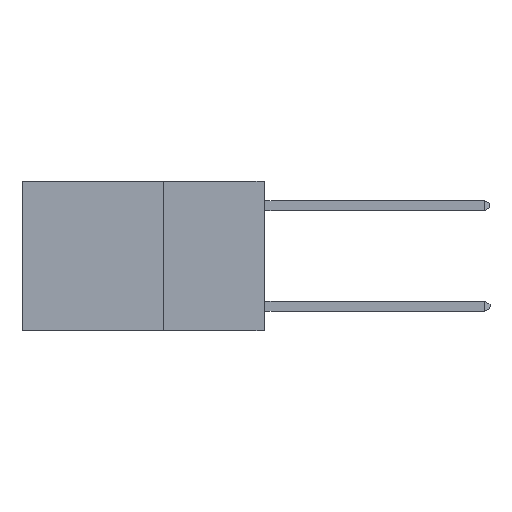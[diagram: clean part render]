
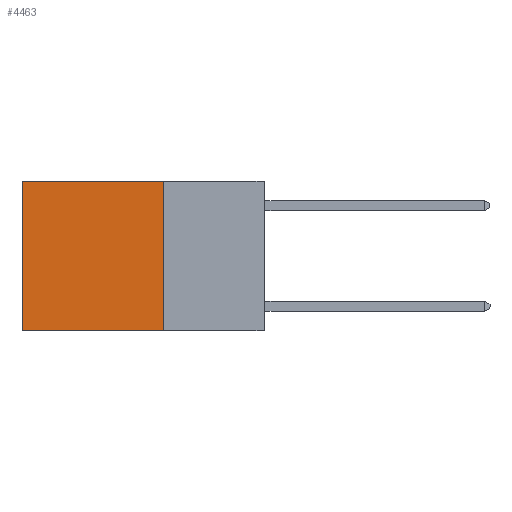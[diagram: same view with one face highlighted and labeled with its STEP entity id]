
A CAD part, left-side view. The second image highlights one B-rep face of the part: STEP entity #4463.
In plain terms, the highlighted planar face has unit normal (-1, 0, 0).
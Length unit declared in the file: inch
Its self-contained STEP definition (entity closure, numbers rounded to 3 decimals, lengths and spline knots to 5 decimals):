
#31 = CARTESIAN_POINT ( 'NONE',  ( 0.2625, 0.25, -0.37 ) ) ;
#682 = ORIENTED_EDGE ( 'NONE', *, *, #9963, .T. ) ;
#707 = ORIENTED_EDGE ( 'NONE', *, *, #8171, .F. ) ;
#733 = CARTESIAN_POINT ( 'NONE',  ( 0.2625, 0.25, 0. ) ) ;
#753 = VERTEX_POINT ( 'NONE', #6637 ) ;
#757 = ORIENTED_EDGE ( 'NONE', *, *, #3633, .F. ) ;
#770 = ORIENTED_EDGE ( 'NONE', *, *, #3584, .T. ) ;
#924 = VERTEX_POINT ( 'NONE', #6483 ) ;
#1167 = EDGE_LOOP ( 'NONE', ( #682, #707, #757, #770 ) ) ;
#1769 = VECTOR ( 'NONE', #9483, 39.37008 ) ;
#1896 = DIRECTION ( 'NONE',  ( 0., 1., 0. ) ) ;
#2438 = CARTESIAN_POINT ( 'NONE',  ( 0.2625, 0.25, -0.37 ) ) ;
#2677 = CARTESIAN_POINT ( 'NONE',  ( 0.2625, 0.25, 0. ) ) ;
#2896 = LINE ( 'NONE', #733, #6989 ) ;
#3584 = EDGE_CURVE ( 'NONE', #10229, #924, #2896, .T. ) ;
#3633 = EDGE_CURVE ( 'NONE', #10229, #8711, #6468, .T. ) ;
#4463 = ADVANCED_FACE ( 'NONE', ( #10144 ), #7268, .F. ) ;
#4851 = DIRECTION ( 'NONE',  ( 0., 0., -1. ) ) ;
#6468 = LINE ( 'NONE', #2677, #1769 ) ;
#6483 = CARTESIAN_POINT ( 'NONE',  ( 0.2625, 0.6, 0. ) ) ;
#6539 = VECTOR ( 'NONE', #7364, 39.37008 ) ;
#6637 = CARTESIAN_POINT ( 'NONE',  ( 0.2625, 0.6, -0.37 ) ) ;
#6989 = VECTOR ( 'NONE', #10958, 39.37008 ) ;
#7089 = VECTOR ( 'NONE', #1896, 39.37008 ) ;
#7268 = PLANE ( 'NONE',  #8068 ) ;
#7332 = LINE ( 'NONE', #31, #7089 ) ;
#7364 = DIRECTION ( 'NONE',  ( 0., 0., -1. ) ) ;
#7868 = CARTESIAN_POINT ( 'NONE',  ( 0.2625, 0.25, 0. ) ) ;
#8068 = AXIS2_PLACEMENT_3D ( 'NONE', #8117, #9740, #4851 ) ;
#8117 = CARTESIAN_POINT ( 'NONE',  ( 0.2625, 0.25, 0. ) ) ;
#8171 = EDGE_CURVE ( 'NONE', #8711, #753, #7332, .T. ) ;
#8209 = CARTESIAN_POINT ( 'NONE',  ( 0.2625, 0.6, 0. ) ) ;
#8711 = VERTEX_POINT ( 'NONE', #2438 ) ;
#9483 = DIRECTION ( 'NONE',  ( 0., 0., -1. ) ) ;
#9740 = DIRECTION ( 'NONE',  ( 1., 0., 0. ) ) ;
#9963 = EDGE_CURVE ( 'NONE', #924, #753, #11084, .T. ) ;
#10144 = FACE_OUTER_BOUND ( 'NONE', #1167, .T. ) ;
#10229 = VERTEX_POINT ( 'NONE', #7868 ) ;
#10958 = DIRECTION ( 'NONE',  ( 0., 1., 0. ) ) ;
#11084 = LINE ( 'NONE', #8209, #6539 ) ;
